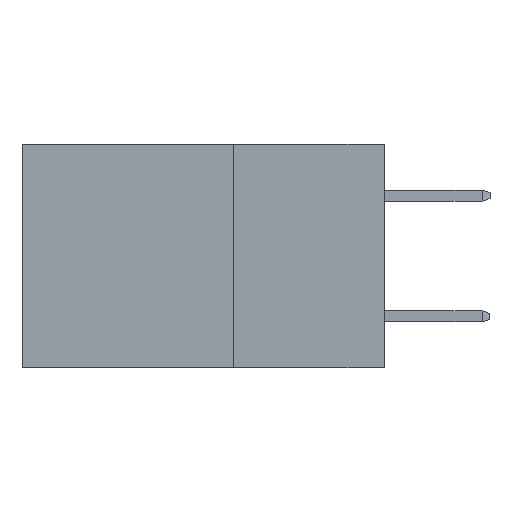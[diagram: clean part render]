
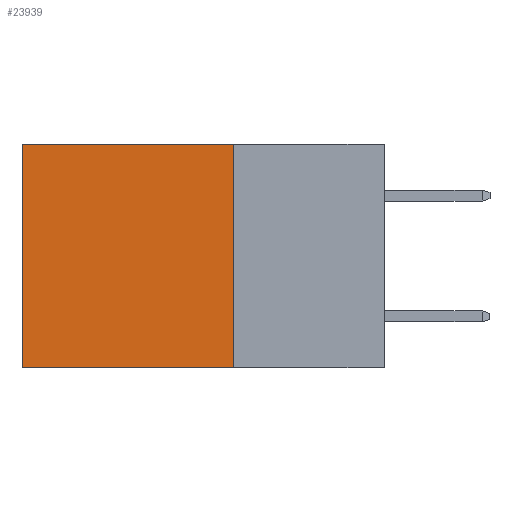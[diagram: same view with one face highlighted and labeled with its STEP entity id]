
A CAD part, left-side view. The second image highlights one B-rep face of the part: STEP entity #23939.
In plain terms, the highlighted planar face has unit normal (-1, 0, 0).
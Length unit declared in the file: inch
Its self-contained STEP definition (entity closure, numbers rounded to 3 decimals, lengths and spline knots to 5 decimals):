
#340 = PLANE ( 'NONE',  #24668 ) ;
#617 = CARTESIAN_POINT ( 'NONE',  ( 0.298, 0.6, -0.37 ) ) ;
#682 = VECTOR ( 'NONE', #11431, 39.37008 ) ;
#2533 = DIRECTION ( 'NONE',  ( 1., 0., 0. ) ) ;
#2672 = VECTOR ( 'NONE', #7306, 39.37008 ) ;
#2788 = EDGE_LOOP ( 'NONE', ( #15242, #21930, #20740, #10512 ) ) ;
#4019 = LINE ( 'NONE', #13690, #20253 ) ;
#4617 = VERTEX_POINT ( 'NONE', #617 ) ;
#5935 = VERTEX_POINT ( 'NONE', #17216 ) ;
#6991 = CARTESIAN_POINT ( 'NONE',  ( 0.298, 0.25, -0.37 ) ) ;
#7306 = DIRECTION ( 'NONE',  ( 0., 1., 0. ) ) ;
#7546 = VECTOR ( 'NONE', #26048, 39.37008 ) ;
#8135 = VERTEX_POINT ( 'NONE', #16657 ) ;
#9291 = CARTESIAN_POINT ( 'NONE',  ( 0.298, 0.6, 0. ) ) ;
#9526 = FACE_OUTER_BOUND ( 'NONE', #2788, .T. ) ;
#10512 = ORIENTED_EDGE ( 'NONE', *, *, #15947, .T. ) ;
#10522 = VERTEX_POINT ( 'NONE', #23830 ) ;
#11431 = DIRECTION ( 'NONE',  ( 0., 0., -1. ) ) ;
#12029 = LINE ( 'NONE', #9291, #682 ) ;
#13159 = LINE ( 'NONE', #6991, #7546 ) ;
#13690 = CARTESIAN_POINT ( 'NONE',  ( 0.298, 0.25, 0. ) ) ;
#15242 = ORIENTED_EDGE ( 'NONE', *, *, #22165, .T. ) ;
#15801 = DIRECTION ( 'NONE',  ( 0., 0., -1. ) ) ;
#15947 = EDGE_CURVE ( 'NONE', #5935, #8135, #25214, .T. ) ;
#16657 = CARTESIAN_POINT ( 'NONE',  ( 0.298, 0.6, 0. ) ) ;
#17216 = CARTESIAN_POINT ( 'NONE',  ( 0.298, 0.25, 0. ) ) ;
#17339 = DIRECTION ( 'NONE',  ( 0., 0., -1. ) ) ;
#19393 = CARTESIAN_POINT ( 'NONE',  ( 0.298, 0.25, 0. ) ) ;
#20253 = VECTOR ( 'NONE', #15801, 39.37008 ) ;
#20740 = ORIENTED_EDGE ( 'NONE', *, *, #22898, .F. ) ;
#21930 = ORIENTED_EDGE ( 'NONE', *, *, #24006, .F. ) ;
#22125 = CARTESIAN_POINT ( 'NONE',  ( 0.298, 0.25, 0. ) ) ;
#22165 = EDGE_CURVE ( 'NONE', #8135, #4617, #12029, .T. ) ;
#22898 = EDGE_CURVE ( 'NONE', #5935, #10522, #4019, .T. ) ;
#23830 = CARTESIAN_POINT ( 'NONE',  ( 0.298, 0.25, -0.37 ) ) ;
#23939 = ADVANCED_FACE ( 'NONE', ( #9526 ), #340, .F. ) ;
#24006 = EDGE_CURVE ( 'NONE', #10522, #4617, #13159, .T. ) ;
#24668 = AXIS2_PLACEMENT_3D ( 'NONE', #19393, #2533, #17339 ) ;
#25214 = LINE ( 'NONE', #22125, #2672 ) ;
#26048 = DIRECTION ( 'NONE',  ( 0., 1., 0. ) ) ;
